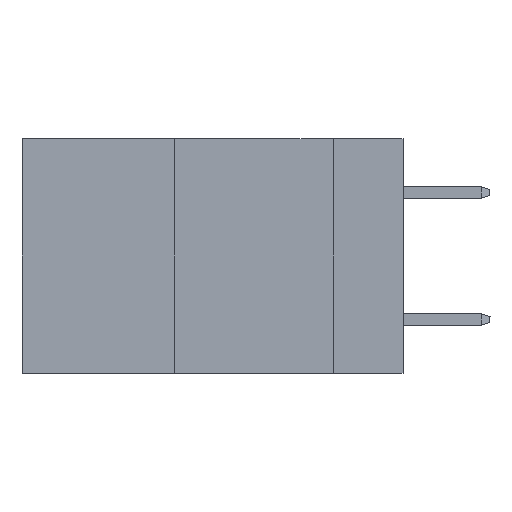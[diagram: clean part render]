
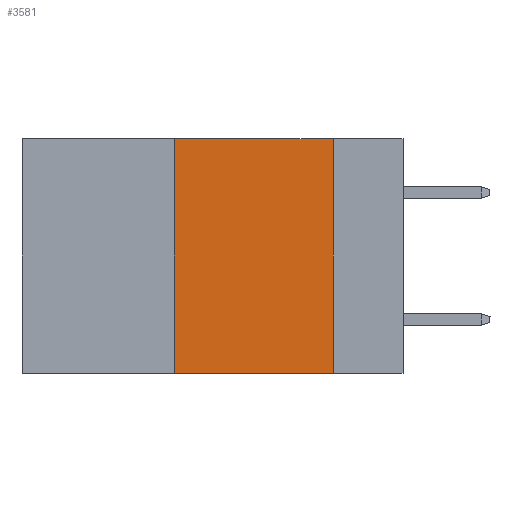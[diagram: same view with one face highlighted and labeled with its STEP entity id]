
A CAD part, left-side view. The second image highlights one B-rep face of the part: STEP entity #3581.
In plain terms, the highlighted planar face has unit normal (-1, 0, 0).
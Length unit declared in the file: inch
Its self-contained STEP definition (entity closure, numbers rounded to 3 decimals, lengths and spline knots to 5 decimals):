
#574 = EDGE_CURVE ( 'NONE', #18586, #13547, #21442, .T. ) ;
#718 = CARTESIAN_POINT ( 'NONE',  ( 0., 0.6, -0.37 ) ) ;
#2481 = EDGE_LOOP ( 'NONE', ( #24108, #7025, #15972, #25879 ) ) ;
#3543 = AXIS2_PLACEMENT_3D ( 'NONE', #22794, #24957, #6425 ) ;
#3581 = ADVANCED_FACE ( 'NONE', ( #14559 ), #6288, .F. ) ;
#3663 = CARTESIAN_POINT ( 'NONE',  ( 0., 0.36, 0. ) ) ;
#4385 = EDGE_CURVE ( 'NONE', #13547, #20612, #6628, .T. ) ;
#4485 = DIRECTION ( 'NONE',  ( 0., 0., -1. ) ) ;
#4569 = EDGE_CURVE ( 'NONE', #23112, #18586, #8454, .T. ) ;
#5897 = VECTOR ( 'NONE', #8608, 39.37008 ) ;
#6288 = PLANE ( 'NONE',  #3543 ) ;
#6425 = DIRECTION ( 'NONE',  ( 0., 0., -1. ) ) ;
#6628 = LINE ( 'NONE', #23398, #10999 ) ;
#7025 = ORIENTED_EDGE ( 'NONE', *, *, #574, .F. ) ;
#8454 = LINE ( 'NONE', #22935, #14900 ) ;
#8608 = DIRECTION ( 'NONE',  ( 0., -1., 0. ) ) ;
#10999 = VECTOR ( 'NONE', #4485, 39.37008 ) ;
#11513 = DIRECTION ( 'NONE',  ( 0., -1., 0. ) ) ;
#13547 = VERTEX_POINT ( 'NONE', #20414 ) ;
#13550 = VECTOR ( 'NONE', #11513, 39.37008 ) ;
#14559 = FACE_OUTER_BOUND ( 'NONE', #2481, .T. ) ;
#14900 = VECTOR ( 'NONE', #25085, 39.37008 ) ;
#15972 = ORIENTED_EDGE ( 'NONE', *, *, #4569, .F. ) ;
#18586 = VERTEX_POINT ( 'NONE', #3663 ) ;
#19431 = EDGE_CURVE ( 'NONE', #23112, #20612, #25821, .T. ) ;
#20414 = CARTESIAN_POINT ( 'NONE',  ( 0., 0.11, 0. ) ) ;
#20612 = VERTEX_POINT ( 'NONE', #25118 ) ;
#21442 = LINE ( 'NONE', #25352, #5897 ) ;
#22794 = CARTESIAN_POINT ( 'NONE',  ( 0., 0.6, 0. ) ) ;
#22935 = CARTESIAN_POINT ( 'NONE',  ( 0., 0.36, 0. ) ) ;
#23112 = VERTEX_POINT ( 'NONE', #26473 ) ;
#23398 = CARTESIAN_POINT ( 'NONE',  ( 0., 0.11, 0. ) ) ;
#24108 = ORIENTED_EDGE ( 'NONE', *, *, #4385, .F. ) ;
#24957 = DIRECTION ( 'NONE',  ( 1., 0., 0. ) ) ;
#25085 = DIRECTION ( 'NONE',  ( 0., 0., 1. ) ) ;
#25118 = CARTESIAN_POINT ( 'NONE',  ( 0., 0.11, -0.37 ) ) ;
#25352 = CARTESIAN_POINT ( 'NONE',  ( 0., 0.6, 0. ) ) ;
#25821 = LINE ( 'NONE', #718, #13550 ) ;
#25879 = ORIENTED_EDGE ( 'NONE', *, *, #19431, .T. ) ;
#26473 = CARTESIAN_POINT ( 'NONE',  ( 0., 0.36, -0.37 ) ) ;
